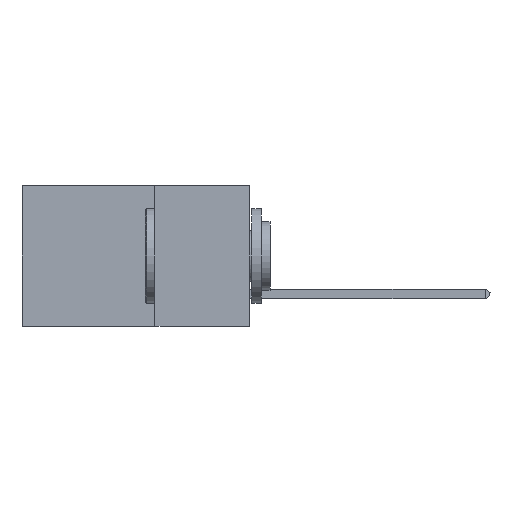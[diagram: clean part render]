
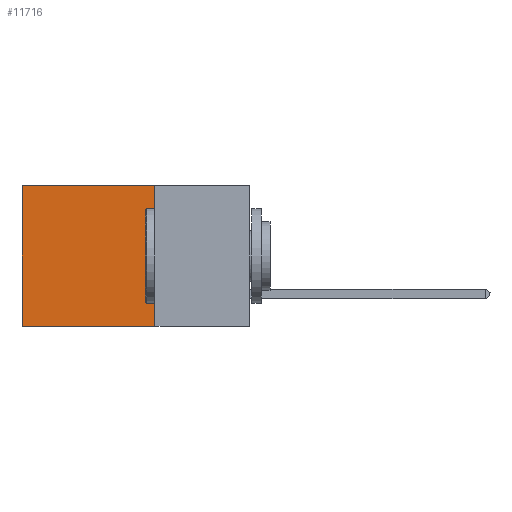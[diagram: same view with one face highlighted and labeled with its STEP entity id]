
A CAD part, left-side view. The second image highlights one B-rep face of the part: STEP entity #11716.
In plain terms, the highlighted planar face has unit normal (-1, 0, 0).
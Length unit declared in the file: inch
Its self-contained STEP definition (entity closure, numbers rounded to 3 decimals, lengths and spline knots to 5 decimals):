
#384 = LINE ( 'NONE', #22835, #4379 ) ;
#1078 = EDGE_CURVE ( 'NONE', #14468, #6958, #384, .T. ) ;
#2078 = VECTOR ( 'NONE', #9926, 39.37008 ) ;
#2101 = VECTOR ( 'NONE', #17648, 39.37008 ) ;
#2200 = CARTESIAN_POINT ( 'NONE',  ( 0.2875, 0.25, 0. ) ) ;
#2384 = VERTEX_POINT ( 'NONE', #16390 ) ;
#4379 = VECTOR ( 'NONE', #17007, 39.37008 ) ;
#5720 = CARTESIAN_POINT ( 'NONE',  ( 0.2875, 0.25, 0. ) ) ;
#6958 = VERTEX_POINT ( 'NONE', #23190 ) ;
#7550 = DIRECTION ( 'NONE',  ( 1., 0., 0. ) ) ;
#8560 = VERTEX_POINT ( 'NONE', #21027 ) ;
#9926 = DIRECTION ( 'NONE',  ( 0., 1., 0. ) ) ;
#11135 = AXIS2_PLACEMENT_3D ( 'NONE', #5720, #7550, #21298 ) ;
#11376 = FACE_OUTER_BOUND ( 'NONE', #22244, .T. ) ;
#11716 = ADVANCED_FACE ( 'NONE', ( #11376 ), #23447, .F. ) ;
#13433 = EDGE_CURVE ( 'NONE', #14468, #8560, #17983, .T. ) ;
#13720 = CARTESIAN_POINT ( 'NONE',  ( 0.2875, 0.6, 0. ) ) ;
#14468 = VERTEX_POINT ( 'NONE', #18054 ) ;
#16390 = CARTESIAN_POINT ( 'NONE',  ( 0.2875, 0.6, -0.37 ) ) ;
#17007 = DIRECTION ( 'NONE',  ( 0., 1., 0. ) ) ;
#17648 = DIRECTION ( 'NONE',  ( 0., 0., -1. ) ) ;
#17752 = LINE ( 'NONE', #13720, #2101 ) ;
#17983 = LINE ( 'NONE', #2200, #24180 ) ;
#18054 = CARTESIAN_POINT ( 'NONE',  ( 0.2875, 0.25, 0. ) ) ;
#18276 = EDGE_CURVE ( 'NONE', #6958, #2384, #17752, .T. ) ;
#19311 = EDGE_CURVE ( 'NONE', #8560, #2384, #23902, .T. ) ;
#21027 = CARTESIAN_POINT ( 'NONE',  ( 0.2875, 0.25, -0.37 ) ) ;
#21298 = DIRECTION ( 'NONE',  ( 0., 0., -1. ) ) ;
#22222 = DIRECTION ( 'NONE',  ( 0., 0., -1. ) ) ;
#22244 = EDGE_LOOP ( 'NONE', ( #24965, #23145, #23667, #22503 ) ) ;
#22503 = ORIENTED_EDGE ( 'NONE', *, *, #1078, .T. ) ;
#22835 = CARTESIAN_POINT ( 'NONE',  ( 0.2875, 0.25, 0. ) ) ;
#23145 = ORIENTED_EDGE ( 'NONE', *, *, #19311, .F. ) ;
#23190 = CARTESIAN_POINT ( 'NONE',  ( 0.2875, 0.6, 0. ) ) ;
#23447 = PLANE ( 'NONE',  #11135 ) ;
#23667 = ORIENTED_EDGE ( 'NONE', *, *, #13433, .F. ) ;
#23902 = LINE ( 'NONE', #25445, #2078 ) ;
#24180 = VECTOR ( 'NONE', #22222, 39.37008 ) ;
#24965 = ORIENTED_EDGE ( 'NONE', *, *, #18276, .T. ) ;
#25445 = CARTESIAN_POINT ( 'NONE',  ( 0.2875, 0.25, -0.37 ) ) ;
